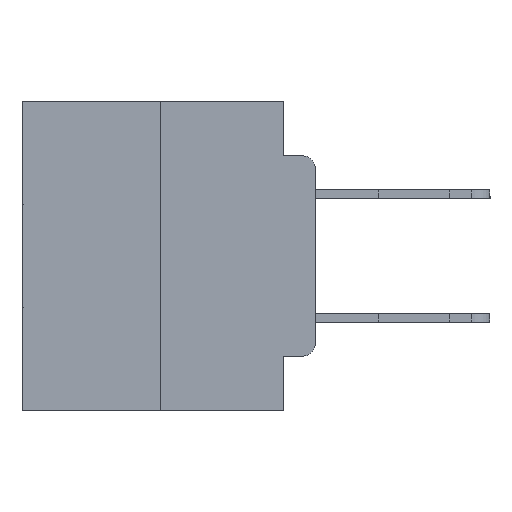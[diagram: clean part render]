
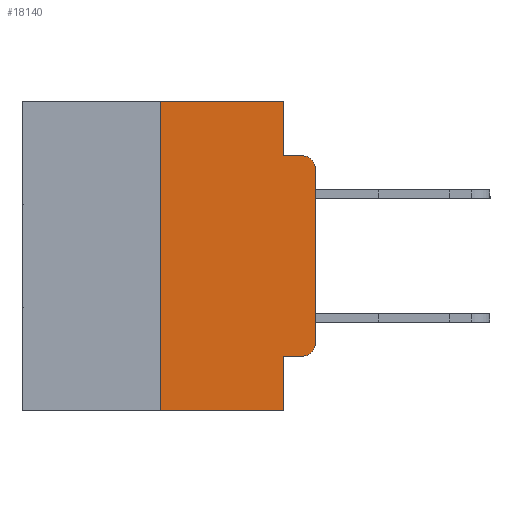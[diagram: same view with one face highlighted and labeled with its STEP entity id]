
A CAD part, left-side view. The second image highlights one B-rep face of the part: STEP entity #18140.
In plain terms, the highlighted planar face has unit normal (-1, 0, 0).
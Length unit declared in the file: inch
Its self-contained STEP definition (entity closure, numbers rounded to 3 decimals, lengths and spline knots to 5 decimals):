
#666 = DIRECTION ( 'NONE',  ( 0., 0., -1. ) ) ;
#858 = CARTESIAN_POINT ( 'NONE',  ( 0., 0.02, -0.4115 ) ) ;
#1067 = VECTOR ( 'NONE', #25085, 39.37008 ) ;
#1129 = ORIENTED_EDGE ( 'NONE', *, *, #18984, .T. ) ;
#1594 = CIRCLE ( 'NONE', #7824, 0.02 ) ;
#1913 = VECTOR ( 'NONE', #9425, 39.37008 ) ;
#1928 = EDGE_CURVE ( 'NONE', #10577, #10618, #15311, .T. ) ;
#1973 = VECTOR ( 'NONE', #5718, 39.37008 ) ;
#2150 = LINE ( 'NONE', #2511, #2900 ) ;
#2425 = VERTEX_POINT ( 'NONE', #3006 ) ;
#2511 = CARTESIAN_POINT ( 'NONE',  ( 0., 0.473, 0. ) ) ;
#2900 = VECTOR ( 'NONE', #14123, 39.37008 ) ;
#3006 = CARTESIAN_POINT ( 'NONE',  ( 0., 0.02, -0.0885 ) ) ;
#3064 = CARTESIAN_POINT ( 'NONE',  ( 0., 0.473, 0. ) ) ;
#3404 = ORIENTED_EDGE ( 'NONE', *, *, #13766, .T. ) ;
#3672 = LINE ( 'NONE', #19374, #27669 ) ;
#4314 = EDGE_CURVE ( 'NONE', #27444, #2425, #11519, .T. ) ;
#4982 = DIRECTION ( 'NONE',  ( -1., 0., 0. ) ) ;
#5585 = DIRECTION ( 'NONE',  ( 0., 0., -1. ) ) ;
#5718 = DIRECTION ( 'NONE',  ( 0., -1., 0. ) ) ;
#5971 = ORIENTED_EDGE ( 'NONE', *, *, #4314, .F. ) ;
#7262 = ORIENTED_EDGE ( 'NONE', *, *, #16688, .F. ) ;
#7824 = AXIS2_PLACEMENT_3D ( 'NONE', #18913, #4982, #21208 ) ;
#7853 = CARTESIAN_POINT ( 'NONE',  ( 0., 0.051, 0. ) ) ;
#8079 = VECTOR ( 'NONE', #5585, 39.37008 ) ;
#9052 = EDGE_CURVE ( 'NONE', #18274, #27444, #3672, .T. ) ;
#9072 = VERTEX_POINT ( 'NONE', #858 ) ;
#9345 = CIRCLE ( 'NONE', #18397, 0.02 ) ;
#9425 = DIRECTION ( 'NONE',  ( 0., -1., 0. ) ) ;
#10070 = DIRECTION ( 'NONE',  ( 0., 0., -1. ) ) ;
#10116 = ORIENTED_EDGE ( 'NONE', *, *, #9052, .F. ) ;
#10278 = CARTESIAN_POINT ( 'NONE',  ( 0., 0.051, -0.4115 ) ) ;
#10577 = VERTEX_POINT ( 'NONE', #17336 ) ;
#10618 = VERTEX_POINT ( 'NONE', #24424 ) ;
#11362 = CARTESIAN_POINT ( 'NONE',  ( 0., 0.25, 0. ) ) ;
#11519 = LINE ( 'NONE', #25937, #29311 ) ;
#13381 = FACE_OUTER_BOUND ( 'NONE', #19145, .T. ) ;
#13622 = VERTEX_POINT ( 'NONE', #14573 ) ;
#13735 = VERTEX_POINT ( 'NONE', #10278 ) ;
#13766 = EDGE_CURVE ( 'NONE', #10577, #18957, #25981, .T. ) ;
#14123 = DIRECTION ( 'NONE',  ( 0., -1., 0. ) ) ;
#14528 = ORIENTED_EDGE ( 'NONE', *, *, #1928, .F. ) ;
#14573 = CARTESIAN_POINT ( 'NONE',  ( 0., 0., -0.1085 ) ) ;
#14605 = DIRECTION ( 'NONE',  ( -1., 0., 0. ) ) ;
#14669 = EDGE_CURVE ( 'NONE', #13735, #9072, #28101, .T. ) ;
#14924 = ORIENTED_EDGE ( 'NONE', *, *, #14669, .T. ) ;
#15311 = LINE ( 'NONE', #11362, #26919 ) ;
#16499 = EDGE_CURVE ( 'NONE', #17122, #13622, #19624, .T. ) ;
#16688 = EDGE_CURVE ( 'NONE', #10618, #18274, #2150, .T. ) ;
#17122 = VERTEX_POINT ( 'NONE', #25047 ) ;
#17336 = CARTESIAN_POINT ( 'NONE',  ( 0., 0.25, -0.5 ) ) ;
#17362 = CARTESIAN_POINT ( 'NONE',  ( 0., 0.051, 0. ) ) ;
#18140 = ADVANCED_FACE ( 'NONE', ( #13381 ), #23872, .F. ) ;
#18274 = VERTEX_POINT ( 'NONE', #17362 ) ;
#18397 = AXIS2_PLACEMENT_3D ( 'NONE', #28516, #14605, #666 ) ;
#18913 = CARTESIAN_POINT ( 'NONE',  ( 0., 0.02, -0.1085 ) ) ;
#18957 = VERTEX_POINT ( 'NONE', #19084 ) ;
#18984 = EDGE_CURVE ( 'NONE', #9072, #17122, #9345, .T. ) ;
#19084 = CARTESIAN_POINT ( 'NONE',  ( 0., 0.051, -0.5 ) ) ;
#19145 = EDGE_LOOP ( 'NONE', ( #29552, #28905, #5971, #10116, #7262, #14528, #3404, #20611, #14924, #1129 ) ) ;
#19374 = CARTESIAN_POINT ( 'NONE',  ( 0., 0.051, 0. ) ) ;
#19624 = LINE ( 'NONE', #24986, #1067 ) ;
#19633 = CARTESIAN_POINT ( 'NONE',  ( 0., 0.473, -0.5 ) ) ;
#20256 = EDGE_CURVE ( 'NONE', #13735, #18957, #26608, .T. ) ;
#20523 = DIRECTION ( 'NONE',  ( 0., 0., 1. ) ) ;
#20611 = ORIENTED_EDGE ( 'NONE', *, *, #20256, .F. ) ;
#20979 = CARTESIAN_POINT ( 'NONE',  ( 0., 0.051, -0.4115 ) ) ;
#21208 = DIRECTION ( 'NONE',  ( 0., 0., -1. ) ) ;
#23872 = PLANE ( 'NONE',  #27906 ) ;
#23961 = DIRECTION ( 'NONE',  ( 1., 0., 0. ) ) ;
#24009 = DIRECTION ( 'NONE',  ( 0., 0., -1. ) ) ;
#24424 = CARTESIAN_POINT ( 'NONE',  ( 0., 0.25, 0. ) ) ;
#24986 = CARTESIAN_POINT ( 'NONE',  ( 0., 0., 0. ) ) ;
#25047 = CARTESIAN_POINT ( 'NONE',  ( 0., 0., -0.3915 ) ) ;
#25085 = DIRECTION ( 'NONE',  ( 0., 0., 1. ) ) ;
#25481 = EDGE_CURVE ( 'NONE', #13622, #2425, #1594, .T. ) ;
#25937 = CARTESIAN_POINT ( 'NONE',  ( 0., 0.051, -0.0885 ) ) ;
#25981 = LINE ( 'NONE', #19633, #1973 ) ;
#26608 = LINE ( 'NONE', #7853, #8079 ) ;
#26919 = VECTOR ( 'NONE', #20523, 39.37008 ) ;
#27444 = VERTEX_POINT ( 'NONE', #29189 ) ;
#27535 = DIRECTION ( 'NONE',  ( 0., -1., 0. ) ) ;
#27669 = VECTOR ( 'NONE', #24009, 39.37008 ) ;
#27906 = AXIS2_PLACEMENT_3D ( 'NONE', #3064, #23961, #10070 ) ;
#28101 = LINE ( 'NONE', #20979, #1913 ) ;
#28516 = CARTESIAN_POINT ( 'NONE',  ( 0., 0.02, -0.3915 ) ) ;
#28905 = ORIENTED_EDGE ( 'NONE', *, *, #25481, .T. ) ;
#29189 = CARTESIAN_POINT ( 'NONE',  ( 0., 0.051, -0.0885 ) ) ;
#29311 = VECTOR ( 'NONE', #27535, 39.37008 ) ;
#29552 = ORIENTED_EDGE ( 'NONE', *, *, #16499, .T. ) ;
